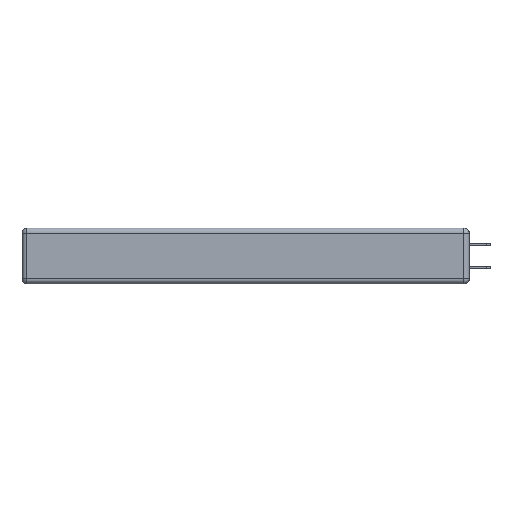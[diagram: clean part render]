
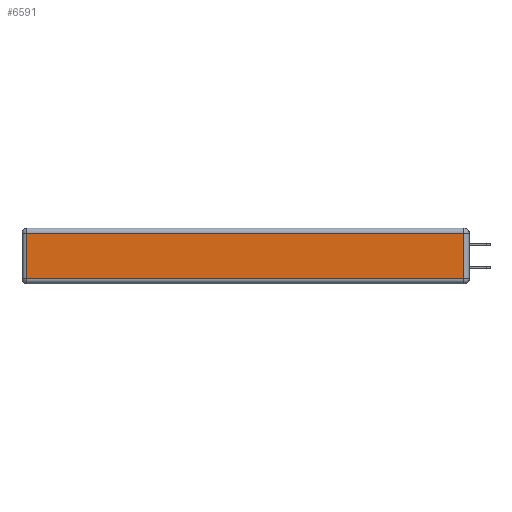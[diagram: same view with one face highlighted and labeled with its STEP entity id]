
A CAD part, left-side view. The second image highlights one B-rep face of the part: STEP entity #6591.
In plain terms, the highlighted planar face has unit normal (-1, 0, 0).
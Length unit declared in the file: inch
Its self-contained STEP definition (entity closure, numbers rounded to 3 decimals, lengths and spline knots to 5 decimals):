
#95 = ORIENTED_EDGE ( 'NONE', *, *, #9596, .T. ) ;
#246 = EDGE_CURVE ( 'NONE', #2121, #11885, #9995, .T. ) ;
#849 = CARTESIAN_POINT ( 'NONE',  ( 0., 2.72, -0.313 ) ) ;
#1065 = PLANE ( 'NONE',  #3879 ) ;
#1800 = CARTESIAN_POINT ( 'NONE',  ( 0., 2.72, -0.03 ) ) ;
#1923 = CARTESIAN_POINT ( 'NONE',  ( 0., 0.03, -0.03 ) ) ;
#2121 = VERTEX_POINT ( 'NONE', #1923 ) ;
#2286 = CARTESIAN_POINT ( 'NONE',  ( 0., 0., -0.313 ) ) ;
#2369 = LINE ( 'NONE', #13214, #13052 ) ;
#2515 = CARTESIAN_POINT ( 'NONE',  ( 0., 2.72, -0.343 ) ) ;
#2937 = LINE ( 'NONE', #2515, #12737 ) ;
#3879 = AXIS2_PLACEMENT_3D ( 'NONE', #12280, #13401, #6697 ) ;
#4172 = VECTOR ( 'NONE', #14462, 39.37008 ) ;
#4562 = DIRECTION ( 'NONE',  ( 0., -1., 0. ) ) ;
#5661 = CARTESIAN_POINT ( 'NONE',  ( 0., 0.03, -0.313 ) ) ;
#6591 = ADVANCED_FACE ( 'NONE', ( #10697 ), #1065, .T. ) ;
#6593 = LINE ( 'NONE', #2286, #9388 ) ;
#6697 = DIRECTION ( 'NONE',  ( 0., 0., 1. ) ) ;
#6814 = VERTEX_POINT ( 'NONE', #849 ) ;
#7811 = EDGE_CURVE ( 'NONE', #11885, #6814, #2937, .T. ) ;
#7995 = ORIENTED_EDGE ( 'NONE', *, *, #7811, .T. ) ;
#8873 = CARTESIAN_POINT ( 'NONE',  ( 0., 2.75, -0.03 ) ) ;
#8948 = EDGE_CURVE ( 'NONE', #6814, #10773, #6593, .T. ) ;
#9204 = ORIENTED_EDGE ( 'NONE', *, *, #246, .T. ) ;
#9388 = VECTOR ( 'NONE', #4562, 39.37008 ) ;
#9596 = EDGE_CURVE ( 'NONE', #10773, #2121, #2369, .T. ) ;
#9995 = LINE ( 'NONE', #8873, #4172 ) ;
#10512 = ORIENTED_EDGE ( 'NONE', *, *, #8948, .T. ) ;
#10697 = FACE_OUTER_BOUND ( 'NONE', #13928, .T. ) ;
#10773 = VERTEX_POINT ( 'NONE', #5661 ) ;
#11341 = DIRECTION ( 'NONE',  ( 0., 0., -1. ) ) ;
#11885 = VERTEX_POINT ( 'NONE', #1800 ) ;
#12280 = CARTESIAN_POINT ( 'NONE',  ( 0., 0., -0.343 ) ) ;
#12737 = VECTOR ( 'NONE', #11341, 39.37008 ) ;
#13052 = VECTOR ( 'NONE', #14357, 39.37008 ) ;
#13214 = CARTESIAN_POINT ( 'NONE',  ( 0., 0.03, -0.343 ) ) ;
#13401 = DIRECTION ( 'NONE',  ( -1., 0., 0. ) ) ;
#13928 = EDGE_LOOP ( 'NONE', ( #10512, #95, #9204, #7995 ) ) ;
#14357 = DIRECTION ( 'NONE',  ( 0., 0., 1. ) ) ;
#14462 = DIRECTION ( 'NONE',  ( 0., 1., 0. ) ) ;
